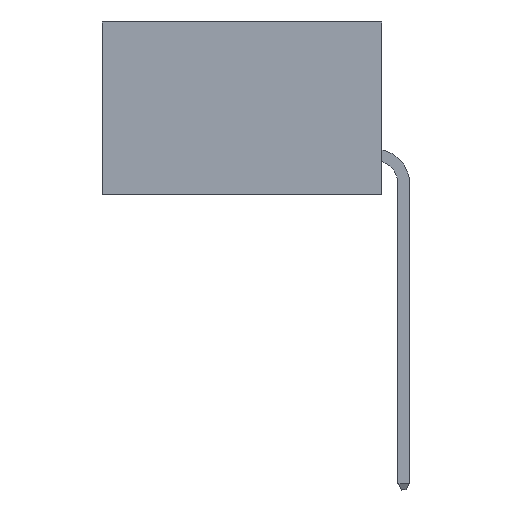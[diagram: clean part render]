
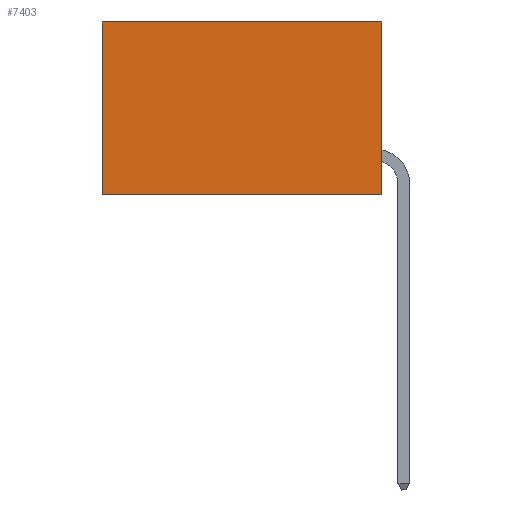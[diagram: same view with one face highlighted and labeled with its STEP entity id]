
A CAD part, left-side view. The second image highlights one B-rep face of the part: STEP entity #7403.
In plain terms, the highlighted planar face has unit normal (-1, 0, 0).
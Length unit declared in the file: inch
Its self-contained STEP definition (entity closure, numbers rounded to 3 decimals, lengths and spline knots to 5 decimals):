
#790 = CARTESIAN_POINT ( 'NONE',  ( 0.2875, 0., -0.37 ) ) ;
#1020 = EDGE_CURVE ( 'NONE', #7829, #2949, #4606, .T. ) ;
#2810 = EDGE_CURVE ( 'NONE', #10642, #2949, #10089, .T. ) ;
#2884 = ORIENTED_EDGE ( 'NONE', *, *, #3100, .T. ) ;
#2948 = VECTOR ( 'NONE', #12498, 39.37008 ) ;
#2949 = VERTEX_POINT ( 'NONE', #10520 ) ;
#2984 = EDGE_LOOP ( 'NONE', ( #10923, #13470, #12604, #2884 ) ) ;
#3100 = EDGE_CURVE ( 'NONE', #4953, #7829, #5103, .T. ) ;
#4339 = DIRECTION ( 'NONE',  ( 0., 1., 0. ) ) ;
#4606 = LINE ( 'NONE', #6599, #14767 ) ;
#4953 = VERTEX_POINT ( 'NONE', #10645 ) ;
#5103 = LINE ( 'NONE', #10812, #8992 ) ;
#5584 = EDGE_CURVE ( 'NONE', #4953, #10642, #9585, .T. ) ;
#5837 = CARTESIAN_POINT ( 'NONE',  ( 0.2875, 0., 0. ) ) ;
#6213 = VECTOR ( 'NONE', #4339, 39.37008 ) ;
#6599 = CARTESIAN_POINT ( 'NONE',  ( 0.2875, 0.6, 0. ) ) ;
#7086 = DIRECTION ( 'NONE',  ( 0., 0., -1. ) ) ;
#7247 = PLANE ( 'NONE',  #8427 ) ;
#7403 = ADVANCED_FACE ( 'NONE', ( #12850 ), #7247, .F. ) ;
#7829 = VERTEX_POINT ( 'NONE', #13716 ) ;
#8059 = DIRECTION ( 'NONE',  ( 0., 0., -1. ) ) ;
#8314 = DIRECTION ( 'NONE',  ( 0., 1., 0. ) ) ;
#8427 = AXIS2_PLACEMENT_3D ( 'NONE', #5837, #14246, #7086 ) ;
#8992 = VECTOR ( 'NONE', #8314, 39.37008 ) ;
#9585 = LINE ( 'NONE', #11297, #2948 ) ;
#10089 = LINE ( 'NONE', #790, #6213 ) ;
#10520 = CARTESIAN_POINT ( 'NONE',  ( 0.2875, 0.6, -0.37 ) ) ;
#10642 = VERTEX_POINT ( 'NONE', #15250 ) ;
#10645 = CARTESIAN_POINT ( 'NONE',  ( 0.2875, 0., 0. ) ) ;
#10812 = CARTESIAN_POINT ( 'NONE',  ( 0.2875, 0., 0. ) ) ;
#10923 = ORIENTED_EDGE ( 'NONE', *, *, #1020, .T. ) ;
#11297 = CARTESIAN_POINT ( 'NONE',  ( 0.2875, 0., 0. ) ) ;
#12498 = DIRECTION ( 'NONE',  ( 0., 0., -1. ) ) ;
#12604 = ORIENTED_EDGE ( 'NONE', *, *, #5584, .F. ) ;
#12850 = FACE_OUTER_BOUND ( 'NONE', #2984, .T. ) ;
#13470 = ORIENTED_EDGE ( 'NONE', *, *, #2810, .F. ) ;
#13716 = CARTESIAN_POINT ( 'NONE',  ( 0.2875, 0.6, 0. ) ) ;
#14246 = DIRECTION ( 'NONE',  ( 1., 0., 0. ) ) ;
#14767 = VECTOR ( 'NONE', #8059, 39.37008 ) ;
#15250 = CARTESIAN_POINT ( 'NONE',  ( 0.2875, 0., -0.37 ) ) ;
